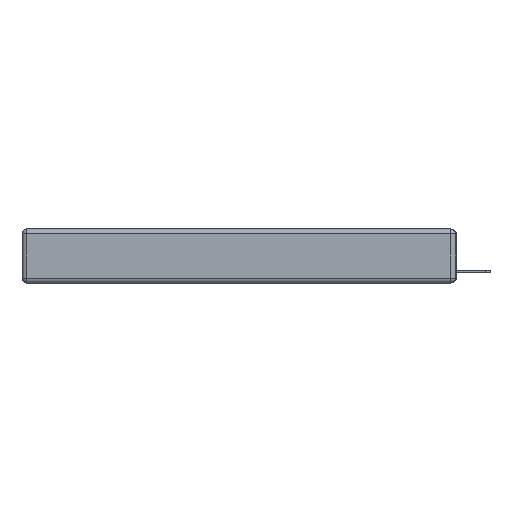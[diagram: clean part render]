
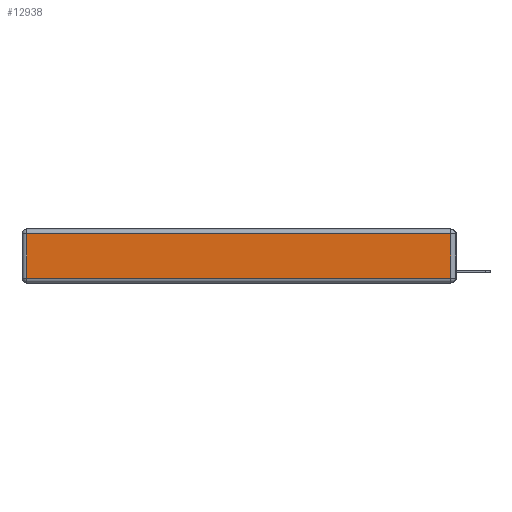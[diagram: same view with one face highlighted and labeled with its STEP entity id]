
A CAD part, left-side view. The second image highlights one B-rep face of the part: STEP entity #12938.
In plain terms, the highlighted planar face has unit normal (-1, 0, 0).
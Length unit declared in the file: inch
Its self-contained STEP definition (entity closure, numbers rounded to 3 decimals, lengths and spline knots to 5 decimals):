
#731 = EDGE_CURVE ( 'NONE', #21106, #8826, #10932, .T. ) ;
#2925 = PLANE ( 'NONE',  #12522 ) ;
#3005 = DIRECTION ( 'NONE',  ( 0., 0., 1. ) ) ;
#3453 = CARTESIAN_POINT ( 'NONE',  ( 0., 0.03, -0.03 ) ) ;
#3658 = CARTESIAN_POINT ( 'NONE',  ( 0., 0.03, -0.313 ) ) ;
#4333 = ORIENTED_EDGE ( 'NONE', *, *, #4416, .T. ) ;
#4416 = EDGE_CURVE ( 'NONE', #8826, #14826, #14124, .T. ) ;
#4492 = VECTOR ( 'NONE', #21298, 39.37008 ) ;
#5145 = LINE ( 'NONE', #11238, #8540 ) ;
#5490 = VERTEX_POINT ( 'NONE', #3453 ) ;
#5850 = DIRECTION ( 'NONE',  ( 0., 0., 1. ) ) ;
#6660 = VECTOR ( 'NONE', #9426, 39.37008 ) ;
#7744 = FACE_OUTER_BOUND ( 'NONE', #11536, .T. ) ;
#8280 = VECTOR ( 'NONE', #19528, 39.37008 ) ;
#8540 = VECTOR ( 'NONE', #5850, 39.37008 ) ;
#8561 = LINE ( 'NONE', #14054, #8280 ) ;
#8826 = VERTEX_POINT ( 'NONE', #12714 ) ;
#9426 = DIRECTION ( 'NONE',  ( 0., 0., -1. ) ) ;
#10932 = LINE ( 'NONE', #18146, #6660 ) ;
#11238 = CARTESIAN_POINT ( 'NONE',  ( 0., 0.03, -0.343 ) ) ;
#11536 = EDGE_LOOP ( 'NONE', ( #4333, #21563, #16934, #12055 ) ) ;
#12055 = ORIENTED_EDGE ( 'NONE', *, *, #731, .T. ) ;
#12522 = AXIS2_PLACEMENT_3D ( 'NONE', #15571, #13831, #3005 ) ;
#12714 = CARTESIAN_POINT ( 'NONE',  ( 0., 2.72, -0.313 ) ) ;
#12938 = ADVANCED_FACE ( 'NONE', ( #7744 ), #2925, .T. ) ;
#13831 = DIRECTION ( 'NONE',  ( -1., 0., 0. ) ) ;
#13911 = EDGE_CURVE ( 'NONE', #5490, #21106, #8561, .T. ) ;
#14054 = CARTESIAN_POINT ( 'NONE',  ( 0., 2.75, -0.03 ) ) ;
#14124 = LINE ( 'NONE', #14179, #4492 ) ;
#14179 = CARTESIAN_POINT ( 'NONE',  ( 0., 0., -0.313 ) ) ;
#14472 = CARTESIAN_POINT ( 'NONE',  ( 0., 2.72, -0.03 ) ) ;
#14826 = VERTEX_POINT ( 'NONE', #3658 ) ;
#15571 = CARTESIAN_POINT ( 'NONE',  ( 0., 0., -0.343 ) ) ;
#16934 = ORIENTED_EDGE ( 'NONE', *, *, #13911, .T. ) ;
#18146 = CARTESIAN_POINT ( 'NONE',  ( 0., 2.72, -0.343 ) ) ;
#19528 = DIRECTION ( 'NONE',  ( 0., 1., 0. ) ) ;
#20533 = EDGE_CURVE ( 'NONE', #14826, #5490, #5145, .T. ) ;
#21106 = VERTEX_POINT ( 'NONE', #14472 ) ;
#21298 = DIRECTION ( 'NONE',  ( 0., -1., 0. ) ) ;
#21563 = ORIENTED_EDGE ( 'NONE', *, *, #20533, .T. ) ;
